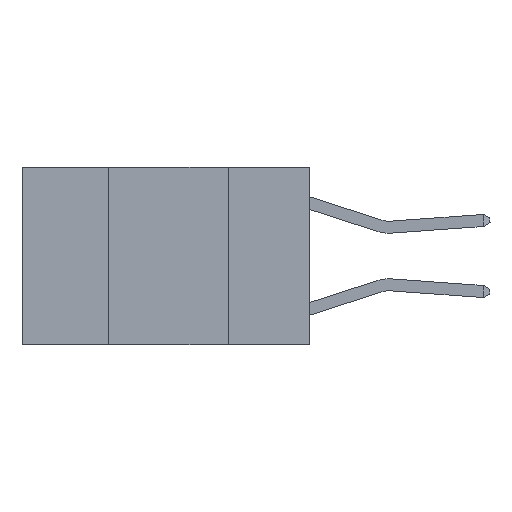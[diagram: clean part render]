
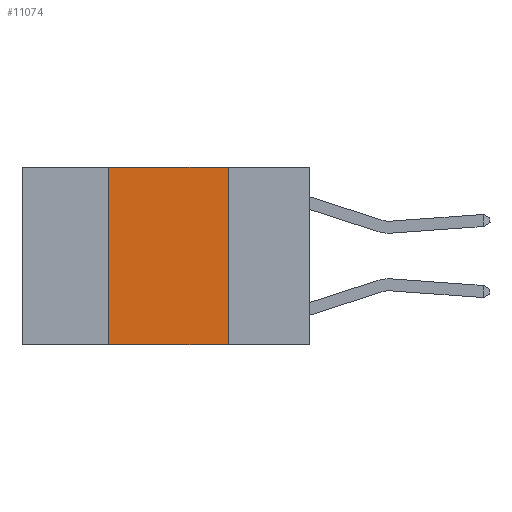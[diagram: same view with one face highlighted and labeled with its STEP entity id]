
A CAD part, left-side view. The second image highlights one B-rep face of the part: STEP entity #11074.
In plain terms, the highlighted planar face has unit normal (-1, 0, 0).
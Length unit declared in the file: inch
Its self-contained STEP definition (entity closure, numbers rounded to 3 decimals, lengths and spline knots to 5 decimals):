
#626 = FACE_OUTER_BOUND ( 'NONE', #7153, .T. ) ;
#1231 = DIRECTION ( 'NONE',  ( 0., -1., 0. ) ) ;
#1502 = ORIENTED_EDGE ( 'NONE', *, *, #14643, .T. ) ;
#1720 = VERTEX_POINT ( 'NONE', #6635 ) ;
#2010 = CARTESIAN_POINT ( 'NONE',  ( 0., 0.17, -0.37 ) ) ;
#2625 = CARTESIAN_POINT ( 'NONE',  ( 0., 0.6, 0. ) ) ;
#2798 = EDGE_CURVE ( 'NONE', #5070, #4299, #8119, .T. ) ;
#4108 = LINE ( 'NONE', #11192, #6424 ) ;
#4299 = VERTEX_POINT ( 'NONE', #2010 ) ;
#5070 = VERTEX_POINT ( 'NONE', #10220 ) ;
#6182 = VECTOR ( 'NONE', #8999, 39.37008 ) ;
#6424 = VECTOR ( 'NONE', #8879, 39.37008 ) ;
#6559 = PLANE ( 'NONE',  #8337 ) ;
#6635 = CARTESIAN_POINT ( 'NONE',  ( 0., 0.42, -0.37 ) ) ;
#7153 = EDGE_LOOP ( 'NONE', ( #10861, #11699, #13747, #1502 ) ) ;
#7177 = VECTOR ( 'NONE', #1231, 39.37008 ) ;
#7537 = DIRECTION ( 'NONE',  ( 1., 0., 0. ) ) ;
#7899 = DIRECTION ( 'NONE',  ( 0., 0., -1. ) ) ;
#8049 = CARTESIAN_POINT ( 'NONE',  ( 0., 0.17, 0. ) ) ;
#8119 = LINE ( 'NONE', #8049, #13187 ) ;
#8337 = AXIS2_PLACEMENT_3D ( 'NONE', #14817, #7537, #13677 ) ;
#8836 = LINE ( 'NONE', #8920, #6182 ) ;
#8879 = DIRECTION ( 'NONE',  ( 0., 0., 1. ) ) ;
#8920 = CARTESIAN_POINT ( 'NONE',  ( 0., 0.6, -0.37 ) ) ;
#8999 = DIRECTION ( 'NONE',  ( 0., -1., 0. ) ) ;
#10220 = CARTESIAN_POINT ( 'NONE',  ( 0., 0.17, 0. ) ) ;
#10363 = CARTESIAN_POINT ( 'NONE',  ( 0., 0.42, 0. ) ) ;
#10861 = ORIENTED_EDGE ( 'NONE', *, *, #2798, .F. ) ;
#11074 = ADVANCED_FACE ( 'NONE', ( #626 ), #6559, .F. ) ;
#11192 = CARTESIAN_POINT ( 'NONE',  ( 0., 0.42, 0. ) ) ;
#11415 = VERTEX_POINT ( 'NONE', #10363 ) ;
#11699 = ORIENTED_EDGE ( 'NONE', *, *, #15083, .F. ) ;
#13187 = VECTOR ( 'NONE', #7899, 39.37008 ) ;
#13677 = DIRECTION ( 'NONE',  ( 0., 0., -1. ) ) ;
#13747 = ORIENTED_EDGE ( 'NONE', *, *, #14045, .F. ) ;
#14045 = EDGE_CURVE ( 'NONE', #1720, #11415, #4108, .T. ) ;
#14402 = LINE ( 'NONE', #2625, #7177 ) ;
#14643 = EDGE_CURVE ( 'NONE', #1720, #4299, #8836, .T. ) ;
#14817 = CARTESIAN_POINT ( 'NONE',  ( 0., 0.6, 0. ) ) ;
#15083 = EDGE_CURVE ( 'NONE', #11415, #5070, #14402, .T. ) ;
